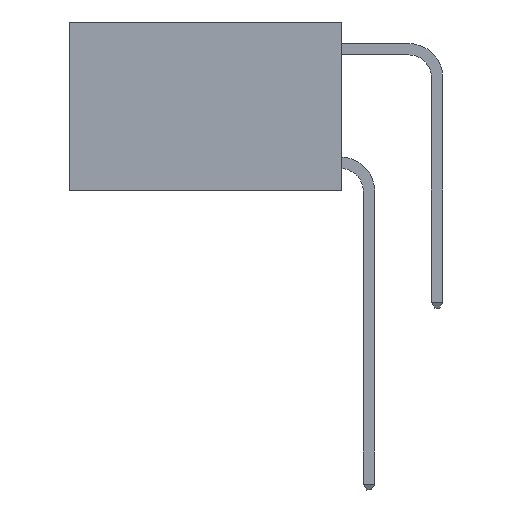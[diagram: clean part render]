
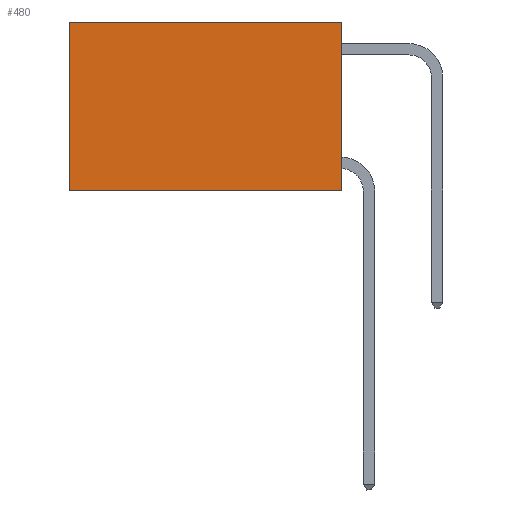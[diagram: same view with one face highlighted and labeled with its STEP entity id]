
A CAD part, left-side view. The second image highlights one B-rep face of the part: STEP entity #480.
In plain terms, the highlighted planar face has unit normal (-1, 0, 0).
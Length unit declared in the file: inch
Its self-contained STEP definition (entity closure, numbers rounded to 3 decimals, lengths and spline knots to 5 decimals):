
#47 = VECTOR ( 'NONE', #6728, 39.37008 ) ;
#257 = ORIENTED_EDGE ( 'NONE', *, *, #10221, .T. ) ;
#466 = EDGE_LOOP ( 'NONE', ( #257, #6992, #561, #5217 ) ) ;
#480 = ADVANCED_FACE ( 'NONE', ( #2391 ), #2924, .F. ) ;
#561 = ORIENTED_EDGE ( 'NONE', *, *, #6319, .F. ) ;
#583 = CARTESIAN_POINT ( 'NONE',  ( 0.2625, 0., 0. ) ) ;
#843 = CARTESIAN_POINT ( 'NONE',  ( 0.2625, 0., -0.37 ) ) ;
#1748 = DIRECTION ( 'NONE',  ( 0., 1., 0. ) ) ;
#1817 = DIRECTION ( 'NONE',  ( 0., 0., -1. ) ) ;
#1830 = DIRECTION ( 'NONE',  ( 1., 0., 0. ) ) ;
#2300 = VECTOR ( 'NONE', #8013, 39.37008 ) ;
#2391 = FACE_OUTER_BOUND ( 'NONE', #466, .T. ) ;
#2424 = AXIS2_PLACEMENT_3D ( 'NONE', #4441, #1830, #1817 ) ;
#2521 = DIRECTION ( 'NONE',  ( 0., 0., -1. ) ) ;
#2529 = VECTOR ( 'NONE', #2521, 39.37008 ) ;
#2582 = EDGE_CURVE ( 'NONE', #9711, #4892, #8617, .T. ) ;
#2700 = VERTEX_POINT ( 'NONE', #6059 ) ;
#2870 = CARTESIAN_POINT ( 'NONE',  ( 0.2625, 0., -0.37 ) ) ;
#2924 = PLANE ( 'NONE',  #2424 ) ;
#3250 = VECTOR ( 'NONE', #1748, 39.37008 ) ;
#3371 = VERTEX_POINT ( 'NONE', #5909 ) ;
#4160 = CARTESIAN_POINT ( 'NONE',  ( 0.2625, 0.6, -0.37 ) ) ;
#4214 = EDGE_CURVE ( 'NONE', #3371, #2700, #5393, .T. ) ;
#4441 = CARTESIAN_POINT ( 'NONE',  ( 0.2625, 0., 0. ) ) ;
#4892 = VERTEX_POINT ( 'NONE', #4160 ) ;
#5217 = ORIENTED_EDGE ( 'NONE', *, *, #4214, .T. ) ;
#5393 = LINE ( 'NONE', #8165, #3250 ) ;
#5909 = CARTESIAN_POINT ( 'NONE',  ( 0.2625, 0., 0. ) ) ;
#6059 = CARTESIAN_POINT ( 'NONE',  ( 0.2625, 0.6, 0. ) ) ;
#6319 = EDGE_CURVE ( 'NONE', #3371, #9711, #8624, .T. ) ;
#6536 = CARTESIAN_POINT ( 'NONE',  ( 0.2625, 0.6, 0. ) ) ;
#6728 = DIRECTION ( 'NONE',  ( 0., 1., 0. ) ) ;
#6992 = ORIENTED_EDGE ( 'NONE', *, *, #2582, .F. ) ;
#7006 = LINE ( 'NONE', #6536, #2529 ) ;
#8013 = DIRECTION ( 'NONE',  ( 0., 0., -1. ) ) ;
#8165 = CARTESIAN_POINT ( 'NONE',  ( 0.2625, 0., 0. ) ) ;
#8617 = LINE ( 'NONE', #843, #47 ) ;
#8624 = LINE ( 'NONE', #583, #2300 ) ;
#9711 = VERTEX_POINT ( 'NONE', #2870 ) ;
#10221 = EDGE_CURVE ( 'NONE', #2700, #4892, #7006, .T. ) ;
